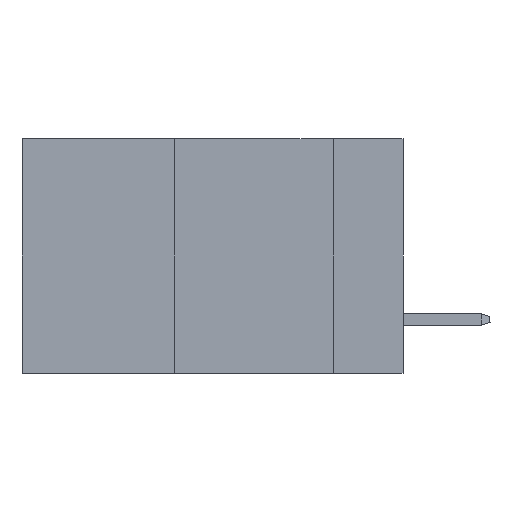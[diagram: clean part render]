
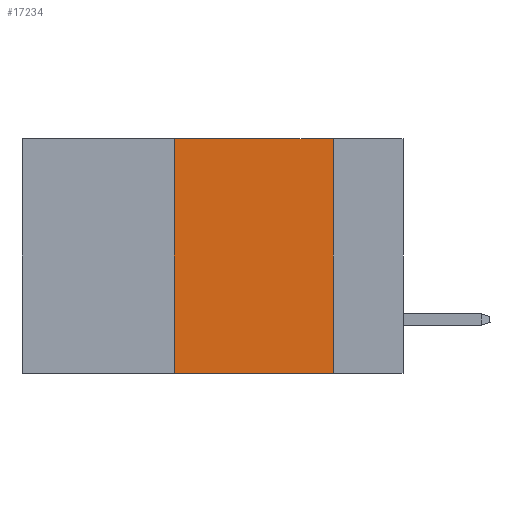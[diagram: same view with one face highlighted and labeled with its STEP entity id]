
A CAD part, left-side view. The second image highlights one B-rep face of the part: STEP entity #17234.
In plain terms, the highlighted planar face has unit normal (-1, 0, 0).
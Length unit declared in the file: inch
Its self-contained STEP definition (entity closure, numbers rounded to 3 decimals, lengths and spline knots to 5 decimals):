
#397 = VERTEX_POINT ( 'NONE', #9441 ) ;
#452 = DIRECTION ( 'NONE',  ( 0., 0., -1. ) ) ;
#1021 = DIRECTION ( 'NONE',  ( 0., -1., 0. ) ) ;
#1552 = VERTEX_POINT ( 'NONE', #17303 ) ;
#3329 = EDGE_CURVE ( 'NONE', #30249, #397, #20340, .T. ) ;
#3857 = CARTESIAN_POINT ( 'NONE',  ( 0., 0.36, 0. ) ) ;
#4164 = LINE ( 'NONE', #15523, #36309 ) ;
#4730 = EDGE_CURVE ( 'NONE', #15559, #1552, #22763, .T. ) ;
#6972 = CARTESIAN_POINT ( 'NONE',  ( 0., 0.6, -0.37 ) ) ;
#7059 = CARTESIAN_POINT ( 'NONE',  ( 0., 0.36, 0. ) ) ;
#7763 = CARTESIAN_POINT ( 'NONE',  ( 0., 0.36, -0.37 ) ) ;
#9441 = CARTESIAN_POINT ( 'NONE',  ( 0., 0.11, 0. ) ) ;
#10575 = EDGE_CURVE ( 'NONE', #15559, #30249, #35017, .T. ) ;
#13425 = EDGE_CURVE ( 'NONE', #397, #1552, #4164, .T. ) ;
#13889 = ORIENTED_EDGE ( 'NONE', *, *, #13425, .F. ) ;
#15523 = CARTESIAN_POINT ( 'NONE',  ( 0., 0.11, 0. ) ) ;
#15559 = VERTEX_POINT ( 'NONE', #7763 ) ;
#16028 = FACE_OUTER_BOUND ( 'NONE', #19394, .T. ) ;
#17234 = ADVANCED_FACE ( 'NONE', ( #16028 ), #37936, .F. ) ;
#17303 = CARTESIAN_POINT ( 'NONE',  ( 0., 0.11, -0.37 ) ) ;
#19394 = EDGE_LOOP ( 'NONE', ( #13889, #24817, #28654, #37192 ) ) ;
#20340 = LINE ( 'NONE', #26503, #39011 ) ;
#21773 = DIRECTION ( 'NONE',  ( 1., 0., 0. ) ) ;
#22763 = LINE ( 'NONE', #6972, #35223 ) ;
#23193 = AXIS2_PLACEMENT_3D ( 'NONE', #28527, #21773, #452 ) ;
#24817 = ORIENTED_EDGE ( 'NONE', *, *, #3329, .F. ) ;
#26503 = CARTESIAN_POINT ( 'NONE',  ( 0., 0.6, 0. ) ) ;
#28527 = CARTESIAN_POINT ( 'NONE',  ( 0., 0.6, 0. ) ) ;
#28654 = ORIENTED_EDGE ( 'NONE', *, *, #10575, .F. ) ;
#30249 = VERTEX_POINT ( 'NONE', #7059 ) ;
#32710 = VECTOR ( 'NONE', #37672, 39.37008 ) ;
#35017 = LINE ( 'NONE', #3857, #32710 ) ;
#35223 = VECTOR ( 'NONE', #1021, 39.37008 ) ;
#35723 = DIRECTION ( 'NONE',  ( 0., 0., -1. ) ) ;
#36098 = DIRECTION ( 'NONE',  ( 0., -1., 0. ) ) ;
#36309 = VECTOR ( 'NONE', #35723, 39.37008 ) ;
#37192 = ORIENTED_EDGE ( 'NONE', *, *, #4730, .T. ) ;
#37672 = DIRECTION ( 'NONE',  ( 0., 0., 1. ) ) ;
#37936 = PLANE ( 'NONE',  #23193 ) ;
#39011 = VECTOR ( 'NONE', #36098, 39.37008 ) ;
